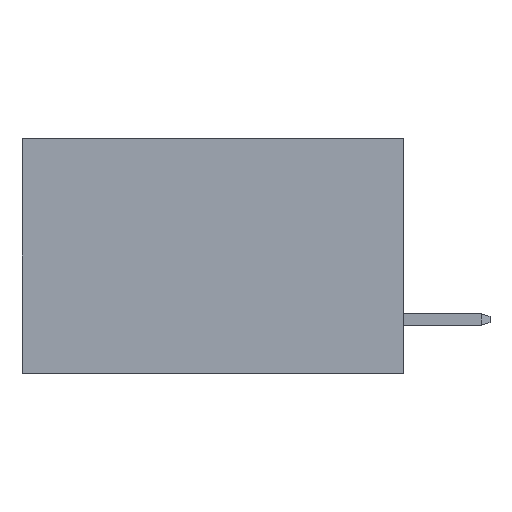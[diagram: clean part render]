
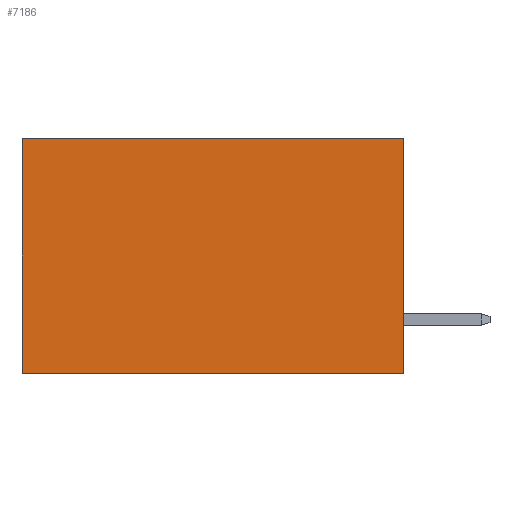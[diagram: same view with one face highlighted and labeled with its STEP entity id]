
A CAD part, left-side view. The second image highlights one B-rep face of the part: STEP entity #7186.
In plain terms, the highlighted planar face has unit normal (-1, 0, 0).
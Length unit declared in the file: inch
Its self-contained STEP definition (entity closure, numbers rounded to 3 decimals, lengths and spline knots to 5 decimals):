
#597 = VERTEX_POINT ( 'NONE', #7118 ) ;
#737 = DIRECTION ( 'NONE',  ( 0., 0., -1. ) ) ;
#1279 = DIRECTION ( 'NONE',  ( 0., 0., -1. ) ) ;
#1326 = CARTESIAN_POINT ( 'NONE',  ( 0.2875, 0., 0. ) ) ;
#2249 = ORIENTED_EDGE ( 'NONE', *, *, #9762, .F. ) ;
#2323 = CARTESIAN_POINT ( 'NONE',  ( 0.2875, 0., 0. ) ) ;
#2427 = EDGE_CURVE ( 'NONE', #9087, #6738, #5933, .T. ) ;
#2759 = PLANE ( 'NONE',  #12185 ) ;
#2772 = CARTESIAN_POINT ( 'NONE',  ( 0.2875, 0.6, -0.37 ) ) ;
#3060 = LINE ( 'NONE', #2323, #6653 ) ;
#3086 = CARTESIAN_POINT ( 'NONE',  ( 0.2875, 0., -0.37 ) ) ;
#3409 = LINE ( 'NONE', #10947, #3532 ) ;
#3532 = VECTOR ( 'NONE', #11128, 39.37008 ) ;
#3755 = CARTESIAN_POINT ( 'NONE',  ( 0.2875, 0., 0. ) ) ;
#4003 = DIRECTION ( 'NONE',  ( 0., 0., -1. ) ) ;
#5014 = EDGE_CURVE ( 'NONE', #5290, #6738, #3409, .T. ) ;
#5290 = VERTEX_POINT ( 'NONE', #3086 ) ;
#5501 = VECTOR ( 'NONE', #1279, 39.37008 ) ;
#5933 = LINE ( 'NONE', #6867, #5501 ) ;
#6653 = VECTOR ( 'NONE', #4003, 39.37008 ) ;
#6738 = VERTEX_POINT ( 'NONE', #2772 ) ;
#6867 = CARTESIAN_POINT ( 'NONE',  ( 0.2875, 0.6, 0. ) ) ;
#6888 = ORIENTED_EDGE ( 'NONE', *, *, #5014, .F. ) ;
#7079 = CARTESIAN_POINT ( 'NONE',  ( 0.2875, 0.6, 0. ) ) ;
#7118 = CARTESIAN_POINT ( 'NONE',  ( 0.2875, 0., 0. ) ) ;
#7186 = ADVANCED_FACE ( 'NONE', ( #11288 ), #2759, .F. ) ;
#8914 = DIRECTION ( 'NONE',  ( 0., 1., 0. ) ) ;
#9087 = VERTEX_POINT ( 'NONE', #7079 ) ;
#9373 = ORIENTED_EDGE ( 'NONE', *, *, #2427, .T. ) ;
#9762 = EDGE_CURVE ( 'NONE', #597, #5290, #3060, .T. ) ;
#9790 = EDGE_CURVE ( 'NONE', #597, #9087, #10728, .T. ) ;
#10416 = DIRECTION ( 'NONE',  ( 1., 0., 0. ) ) ;
#10728 = LINE ( 'NONE', #1326, #11235 ) ;
#10947 = CARTESIAN_POINT ( 'NONE',  ( 0.2875, 0., -0.37 ) ) ;
#11047 = ORIENTED_EDGE ( 'NONE', *, *, #9790, .T. ) ;
#11128 = DIRECTION ( 'NONE',  ( 0., 1., 0. ) ) ;
#11235 = VECTOR ( 'NONE', #8914, 39.37008 ) ;
#11288 = FACE_OUTER_BOUND ( 'NONE', #11385, .T. ) ;
#11385 = EDGE_LOOP ( 'NONE', ( #9373, #6888, #2249, #11047 ) ) ;
#12185 = AXIS2_PLACEMENT_3D ( 'NONE', #3755, #10416, #737 ) ;
